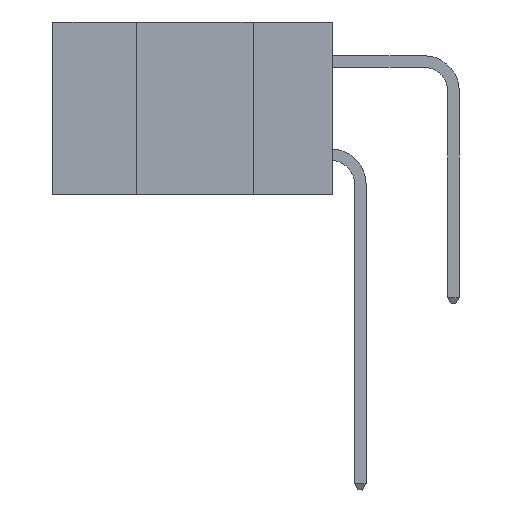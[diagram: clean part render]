
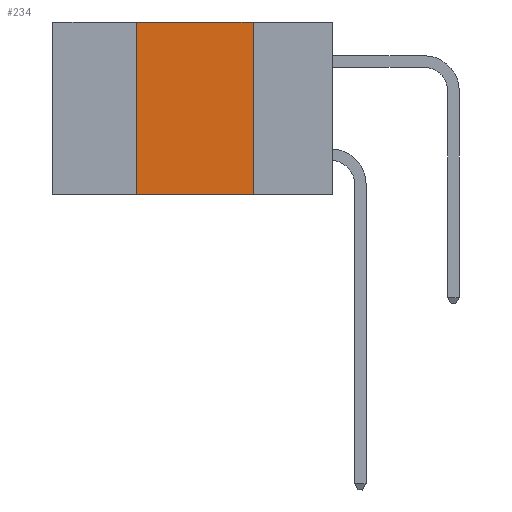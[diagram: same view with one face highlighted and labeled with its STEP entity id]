
A CAD part, left-side view. The second image highlights one B-rep face of the part: STEP entity #234.
In plain terms, the highlighted planar face has unit normal (-1, 0, 0).
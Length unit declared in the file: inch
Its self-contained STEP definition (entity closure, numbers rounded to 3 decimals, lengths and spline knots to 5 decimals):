
#234 = ADVANCED_FACE ( 'NONE', ( #3670 ), #14392, .F. ) ;
#387 = ORIENTED_EDGE ( 'NONE', *, *, #17394, .F. ) ;
#595 = CARTESIAN_POINT ( 'NONE',  ( 0., 0.42, -0.37 ) ) ;
#1076 = VECTOR ( 'NONE', #10571, 39.37008 ) ;
#1428 = LINE ( 'NONE', #2754, #14044 ) ;
#2580 = DIRECTION ( 'NONE',  ( 0., 0., 1. ) ) ;
#2754 = CARTESIAN_POINT ( 'NONE',  ( 0., 0.42, 0. ) ) ;
#3670 = FACE_OUTER_BOUND ( 'NONE', #5663, .T. ) ;
#3761 = CARTESIAN_POINT ( 'NONE',  ( 0., 0.42, 0. ) ) ;
#4070 = LINE ( 'NONE', #11988, #15578 ) ;
#4473 = ORIENTED_EDGE ( 'NONE', *, *, #6065, .F. ) ;
#4793 = ORIENTED_EDGE ( 'NONE', *, *, #15024, .T. ) ;
#5030 = LINE ( 'NONE', #14260, #17358 ) ;
#5057 = CARTESIAN_POINT ( 'NONE',  ( 0., 0.6, 0. ) ) ;
#5663 = EDGE_LOOP ( 'NONE', ( #387, #4473, #11566, #4793 ) ) ;
#6065 = EDGE_CURVE ( 'NONE', #14567, #14379, #13708, .T. ) ;
#7469 = AXIS2_PLACEMENT_3D ( 'NONE', #11737, #17207, #10289 ) ;
#7973 = DIRECTION ( 'NONE',  ( 0., -1., 0. ) ) ;
#8010 = VERTEX_POINT ( 'NONE', #10843 ) ;
#10289 = DIRECTION ( 'NONE',  ( 0., 0., -1. ) ) ;
#10571 = DIRECTION ( 'NONE',  ( 0., -1., 0. ) ) ;
#10843 = CARTESIAN_POINT ( 'NONE',  ( 0., 0.17, -0.37 ) ) ;
#11566 = ORIENTED_EDGE ( 'NONE', *, *, #14123, .F. ) ;
#11737 = CARTESIAN_POINT ( 'NONE',  ( 0., 0.6, 0. ) ) ;
#11988 = CARTESIAN_POINT ( 'NONE',  ( 0., 0.17, 0. ) ) ;
#13370 = DIRECTION ( 'NONE',  ( 0., 0., -1. ) ) ;
#13708 = LINE ( 'NONE', #5057, #1076 ) ;
#14044 = VECTOR ( 'NONE', #2580, 39.37008 ) ;
#14123 = EDGE_CURVE ( 'NONE', #16127, #14567, #1428, .T. ) ;
#14260 = CARTESIAN_POINT ( 'NONE',  ( 0., 0.6, -0.37 ) ) ;
#14379 = VERTEX_POINT ( 'NONE', #16808 ) ;
#14392 = PLANE ( 'NONE',  #7469 ) ;
#14567 = VERTEX_POINT ( 'NONE', #3761 ) ;
#15024 = EDGE_CURVE ( 'NONE', #16127, #8010, #5030, .T. ) ;
#15578 = VECTOR ( 'NONE', #13370, 39.37008 ) ;
#16127 = VERTEX_POINT ( 'NONE', #595 ) ;
#16808 = CARTESIAN_POINT ( 'NONE',  ( 0., 0.17, 0. ) ) ;
#17207 = DIRECTION ( 'NONE',  ( 1., 0., 0. ) ) ;
#17358 = VECTOR ( 'NONE', #7973, 39.37008 ) ;
#17394 = EDGE_CURVE ( 'NONE', #14379, #8010, #4070, .T. ) ;
